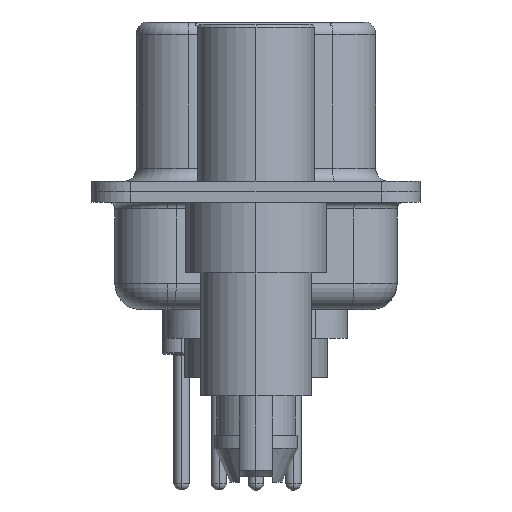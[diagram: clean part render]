
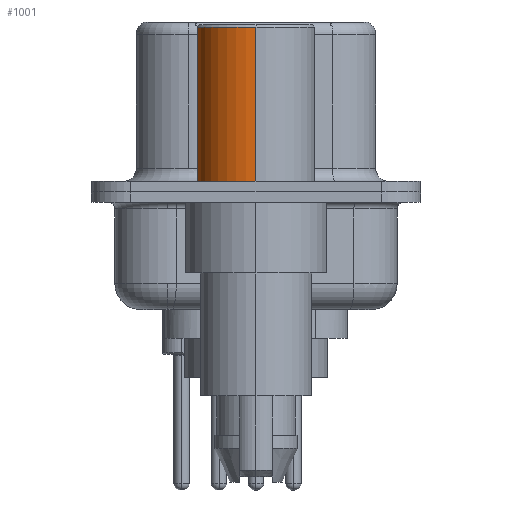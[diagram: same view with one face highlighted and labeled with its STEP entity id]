
A CAD part, left-side view. The second image highlights one B-rep face of the part: STEP entity #1001.
In plain terms, the highlighted cylindrical face has radius 2.25 mm (diameter 4.5 mm), a partial arc.
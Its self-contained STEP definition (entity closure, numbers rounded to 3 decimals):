
#159 = CARTESIAN_POINT ( 'NONE',  ( 2.25, 0., 0.581 ) ) ;
#556 = ORIENTED_EDGE ( 'NONE', *, *, #18604, .T. ) ;
#1001 = ADVANCED_FACE ( 'NONE', ( #3202 ), #2623, .T. ) ;
#1203 = CARTESIAN_POINT ( 'NONE',  ( 2.25, 0., 6.3 ) ) ;
#2243 = VECTOR ( 'NONE', #13027, 1000. ) ;
#2315 = AXIS2_PLACEMENT_3D ( 'NONE', #21101, #10207, #22976 ) ;
#2623 = CYLINDRICAL_SURFACE ( 'NONE', #16948, 2.25 ) ;
#3197 = CARTESIAN_POINT ( 'NONE',  ( 0., 0., 0.4 ) ) ;
#3202 = FACE_OUTER_BOUND ( 'NONE', #19065, .T. ) ;
#4834 = CARTESIAN_POINT ( 'NONE',  ( -2.25, 0., 0.581 ) ) ;
#5122 = DIRECTION ( 'NONE',  ( 1., 0., 0. ) ) ;
#7733 = LINE ( 'NONE', #159, #2243 ) ;
#8069 = CIRCLE ( 'NONE', #9835, 2.25 ) ;
#8740 = VERTEX_POINT ( 'NONE', #11980 ) ;
#9835 = AXIS2_PLACEMENT_3D ( 'NONE', #3197, #15928, #5122 ) ;
#10207 = DIRECTION ( 'NONE',  ( 0., 0., 1. ) ) ;
#10921 = ORIENTED_EDGE ( 'NONE', *, *, #23501, .F. ) ;
#11980 = CARTESIAN_POINT ( 'NONE',  ( -2.25, 0., 6.3 ) ) ;
#11997 = CARTESIAN_POINT ( 'NONE',  ( -2.25, 0., 0.4 ) ) ;
#13027 = DIRECTION ( 'NONE',  ( 0., 0., 1. ) ) ;
#13276 = EDGE_CURVE ( 'NONE', #18405, #17482, #8069, .T. ) ;
#14101 = VECTOR ( 'NONE', #19369, 1000. ) ;
#14532 = ORIENTED_EDGE ( 'NONE', *, *, #13276, .T. ) ;
#15111 = CARTESIAN_POINT ( 'NONE',  ( 2.25, 0., 0.4 ) ) ;
#15128 = DIRECTION ( 'NONE',  ( 1., 0., 0. ) ) ;
#15608 = CIRCLE ( 'NONE', #2315, 2.25 ) ;
#15928 = DIRECTION ( 'NONE',  ( 0., 0., 1. ) ) ;
#16948 = AXIS2_PLACEMENT_3D ( 'NONE', #18690, #19991, #15128 ) ;
#17482 = VERTEX_POINT ( 'NONE', #11997 ) ;
#18405 = VERTEX_POINT ( 'NONE', #15111 ) ;
#18604 = EDGE_CURVE ( 'NONE', #17482, #8740, #18982, .T. ) ;
#18660 = VERTEX_POINT ( 'NONE', #1203 ) ;
#18690 = CARTESIAN_POINT ( 'NONE',  ( 0., 0., 0.581 ) ) ;
#18982 = LINE ( 'NONE', #4834, #14101 ) ;
#19065 = EDGE_LOOP ( 'NONE', ( #14532, #556, #10921, #19233 ) ) ;
#19233 = ORIENTED_EDGE ( 'NONE', *, *, #22842, .F. ) ;
#19369 = DIRECTION ( 'NONE',  ( 0., 0., 1. ) ) ;
#19991 = DIRECTION ( 'NONE',  ( 0., 0., 1. ) ) ;
#21101 = CARTESIAN_POINT ( 'NONE',  ( 0., 0., 6.3 ) ) ;
#22842 = EDGE_CURVE ( 'NONE', #18405, #18660, #7733, .T. ) ;
#22976 = DIRECTION ( 'NONE',  ( 1., 0., 0. ) ) ;
#23501 = EDGE_CURVE ( 'NONE', #18660, #8740, #15608, .T. ) ;
